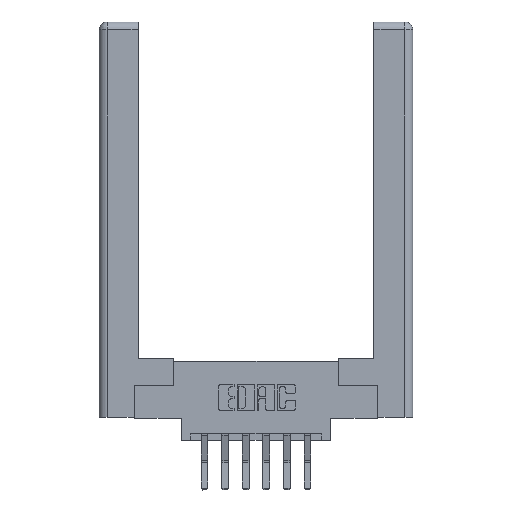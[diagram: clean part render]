
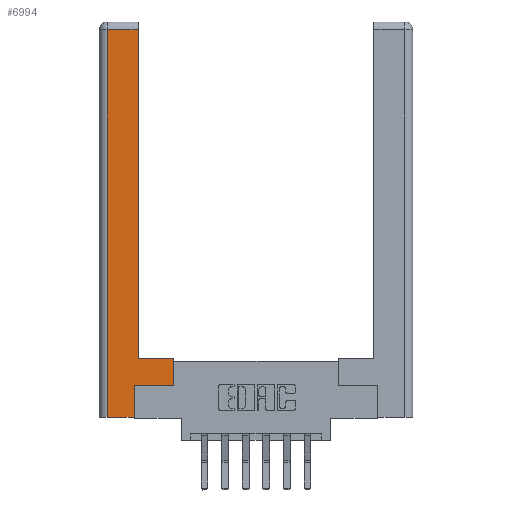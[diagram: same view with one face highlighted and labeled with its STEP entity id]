
A CAD part, top view. The second image highlights one B-rep face of the part: STEP entity #6994.
In plain terms, the highlighted planar face has unit normal (0, 0, 1).
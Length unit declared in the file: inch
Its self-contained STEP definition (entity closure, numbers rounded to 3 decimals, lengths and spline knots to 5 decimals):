
#17 = LINE ( 'NONE', #10258, #7804 ) ;
#41 = VECTOR ( 'NONE', #3399, 39.37008 ) ;
#771 = ORIENTED_EDGE ( 'NONE', *, *, #11614, .T. ) ;
#981 = ORIENTED_EDGE ( 'NONE', *, *, #9927, .T. ) ;
#1070 = ORIENTED_EDGE ( 'NONE', *, *, #2716, .T. ) ;
#1642 = VERTEX_POINT ( 'NONE', #6350 ) ;
#1648 = CARTESIAN_POINT ( 'NONE',  ( 0.265, 0.245, 0. ) ) ;
#1687 = PLANE ( 'NONE',  #7065 ) ;
#1717 = VECTOR ( 'NONE', #10270, 39.37008 ) ;
#1783 = VECTOR ( 'NONE', #7976, 39.37008 ) ;
#2021 = LINE ( 'NONE', #2714, #1717 ) ;
#2419 = VERTEX_POINT ( 'NONE', #8428 ) ;
#2459 = CARTESIAN_POINT ( 'NONE',  ( 0.295, 2.94, 0. ) ) ;
#2472 = DIRECTION ( 'NONE',  ( -1., 0., 0. ) ) ;
#2490 = VECTOR ( 'NONE', #9314, 39.37008 ) ;
#2506 = ORIENTED_EDGE ( 'NONE', *, *, #8753, .T. ) ;
#2513 = LINE ( 'NONE', #5222, #41 ) ;
#2516 = DIRECTION ( 'NONE',  ( 0., 1., 0. ) ) ;
#2714 = CARTESIAN_POINT ( 'NONE',  ( 0.295, 0.45, 0. ) ) ;
#2716 = EDGE_CURVE ( 'NONE', #3692, #3127, #7354, .T. ) ;
#2817 = LINE ( 'NONE', #6568, #11228 ) ;
#3052 = ORIENTED_EDGE ( 'NONE', *, *, #3702, .T. ) ;
#3127 = VERTEX_POINT ( 'NONE', #12156 ) ;
#3399 = DIRECTION ( 'NONE',  ( 0., -1., 0. ) ) ;
#3692 = VERTEX_POINT ( 'NONE', #9363 ) ;
#3702 = EDGE_CURVE ( 'NONE', #6228, #3692, #7652, .T. ) ;
#4324 = EDGE_CURVE ( 'NONE', #9677, #5330, #10633, .T. ) ;
#4539 = CARTESIAN_POINT ( 'NONE',  ( 0.0615, 0., 0. ) ) ;
#4756 = CARTESIAN_POINT ( 'NONE',  ( 0.565, 0.45, 0. ) ) ;
#5222 = CARTESIAN_POINT ( 'NONE',  ( 0.0615, 0., 0. ) ) ;
#5330 = VERTEX_POINT ( 'NONE', #9624 ) ;
#6142 = VECTOR ( 'NONE', #8513, 39.37008 ) ;
#6228 = VERTEX_POINT ( 'NONE', #4539 ) ;
#6350 = CARTESIAN_POINT ( 'NONE',  ( 0.565, 0.45, 0. ) ) ;
#6508 = ORIENTED_EDGE ( 'NONE', *, *, #4324, .T. ) ;
#6568 = CARTESIAN_POINT ( 'NONE',  ( 0.295, 3., 0. ) ) ;
#6994 = ADVANCED_FACE ( 'NONE', ( #8876 ), #1687, .F. ) ;
#7065 = AXIS2_PLACEMENT_3D ( 'NONE', #10147, #7155, #2472 ) ;
#7155 = DIRECTION ( 'NONE',  ( 0., 0., -1. ) ) ;
#7354 = LINE ( 'NONE', #1648, #11496 ) ;
#7390 = CARTESIAN_POINT ( 'NONE',  ( 0.265, 0., 0. ) ) ;
#7652 = LINE ( 'NONE', #7390, #2490 ) ;
#7804 = VECTOR ( 'NONE', #10412, 39.37008 ) ;
#7976 = DIRECTION ( 'NONE',  ( -1., 0., 0. ) ) ;
#8198 = EDGE_CURVE ( 'NONE', #2419, #9677, #2817, .T. ) ;
#8428 = CARTESIAN_POINT ( 'NONE',  ( 0.295, 0.45, 0. ) ) ;
#8513 = DIRECTION ( 'NONE',  ( 0., 1., 0. ) ) ;
#8753 = EDGE_CURVE ( 'NONE', #5330, #6228, #2513, .T. ) ;
#8876 = FACE_OUTER_BOUND ( 'NONE', #9094, .T. ) ;
#9094 = EDGE_LOOP ( 'NONE', ( #10729, #6508, #2506, #3052, #1070, #9159, #981, #771 ) ) ;
#9159 = ORIENTED_EDGE ( 'NONE', *, *, #9255, .T. ) ;
#9255 = EDGE_CURVE ( 'NONE', #3127, #9698, #17, .T. ) ;
#9314 = DIRECTION ( 'NONE',  ( 1., 0., 0. ) ) ;
#9363 = CARTESIAN_POINT ( 'NONE',  ( 0.265, 0., 0. ) ) ;
#9624 = CARTESIAN_POINT ( 'NONE',  ( 0.0615, 2.94, 0. ) ) ;
#9677 = VERTEX_POINT ( 'NONE', #2459 ) ;
#9698 = VERTEX_POINT ( 'NONE', #10099 ) ;
#9880 = CARTESIAN_POINT ( 'NONE',  ( 0.0615, 2.94, 0. ) ) ;
#9927 = EDGE_CURVE ( 'NONE', #9698, #1642, #11470, .T. ) ;
#10099 = CARTESIAN_POINT ( 'NONE',  ( 0.565, 0.245, 0. ) ) ;
#10147 = CARTESIAN_POINT ( 'NONE',  ( 0., 0., 0. ) ) ;
#10258 = CARTESIAN_POINT ( 'NONE',  ( 0.565, 0.245, 0. ) ) ;
#10270 = DIRECTION ( 'NONE',  ( -1., 0., 0. ) ) ;
#10412 = DIRECTION ( 'NONE',  ( 1., 0., 0. ) ) ;
#10419 = DIRECTION ( 'NONE',  ( 0., 1., 0. ) ) ;
#10633 = LINE ( 'NONE', #9880, #1783 ) ;
#10729 = ORIENTED_EDGE ( 'NONE', *, *, #8198, .T. ) ;
#11228 = VECTOR ( 'NONE', #10419, 39.37008 ) ;
#11470 = LINE ( 'NONE', #4756, #6142 ) ;
#11496 = VECTOR ( 'NONE', #2516, 39.37008 ) ;
#11614 = EDGE_CURVE ( 'NONE', #1642, #2419, #2021, .T. ) ;
#12156 = CARTESIAN_POINT ( 'NONE',  ( 0.265, 0.245, 0. ) ) ;
